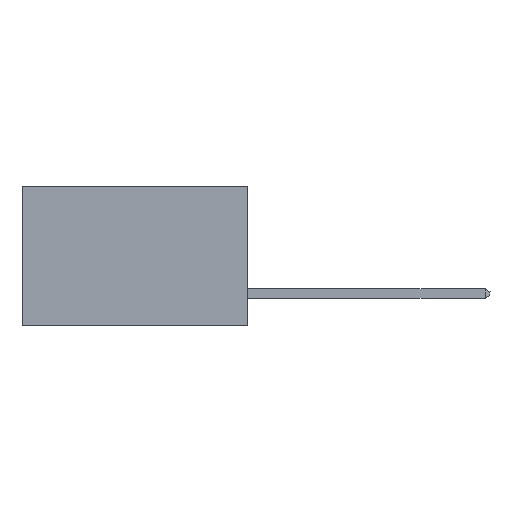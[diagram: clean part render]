
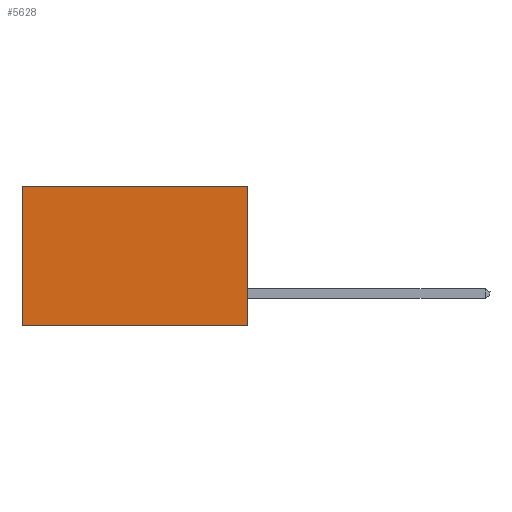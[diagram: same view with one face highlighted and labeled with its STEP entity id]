
A CAD part, left-side view. The second image highlights one B-rep face of the part: STEP entity #5628.
In plain terms, the highlighted planar face has unit normal (-1, 0, 0).
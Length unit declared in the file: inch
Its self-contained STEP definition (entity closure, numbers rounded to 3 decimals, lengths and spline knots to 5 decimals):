
#432 = CARTESIAN_POINT ( 'NONE',  ( 0.2615, 0.6, 0. ) ) ;
#1112 = VERTEX_POINT ( 'NONE', #9807 ) ;
#1156 = ORIENTED_EDGE ( 'NONE', *, *, #6772, .F. ) ;
#1478 = DIRECTION ( 'NONE',  ( 0., 1., 0. ) ) ;
#1571 = LINE ( 'NONE', #8122, #10280 ) ;
#1751 = VERTEX_POINT ( 'NONE', #432 ) ;
#2314 = FACE_OUTER_BOUND ( 'NONE', #3891, .T. ) ;
#2470 = ORIENTED_EDGE ( 'NONE', *, *, #9550, .T. ) ;
#3038 = EDGE_CURVE ( 'NONE', #3798, #1751, #3789, .T. ) ;
#3789 = LINE ( 'NONE', #7687, #6929 ) ;
#3798 = VERTEX_POINT ( 'NONE', #9347 ) ;
#3891 = EDGE_LOOP ( 'NONE', ( #2470, #1156, #8669, #4152 ) ) ;
#4152 = ORIENTED_EDGE ( 'NONE', *, *, #3038, .T. ) ;
#4418 = VERTEX_POINT ( 'NONE', #9647 ) ;
#4523 = DIRECTION ( 'NONE',  ( 0., 1., 0. ) ) ;
#4527 = CARTESIAN_POINT ( 'NONE',  ( 0.2615, 0., -0.37 ) ) ;
#4575 = DIRECTION ( 'NONE',  ( 1., 0., 0. ) ) ;
#4884 = DIRECTION ( 'NONE',  ( 0., 0., -1. ) ) ;
#5257 = LINE ( 'NONE', #5948, #5365 ) ;
#5365 = VECTOR ( 'NONE', #8401, 39.37008 ) ;
#5488 = VECTOR ( 'NONE', #1478, 39.37008 ) ;
#5628 = ADVANCED_FACE ( 'NONE', ( #2314 ), #6374, .F. ) ;
#5674 = CARTESIAN_POINT ( 'NONE',  ( 0.2615, 0., -0.37 ) ) ;
#5948 = CARTESIAN_POINT ( 'NONE',  ( 0.2615, 0.6, -0.37 ) ) ;
#6209 = DIRECTION ( 'NONE',  ( 0., 0., -1. ) ) ;
#6374 = PLANE ( 'NONE',  #9837 ) ;
#6377 = LINE ( 'NONE', #5674, #5488 ) ;
#6772 = EDGE_CURVE ( 'NONE', #4418, #1112, #6377, .T. ) ;
#6929 = VECTOR ( 'NONE', #4523, 39.37008 ) ;
#7687 = CARTESIAN_POINT ( 'NONE',  ( 0.2615, 0., 0. ) ) ;
#8122 = CARTESIAN_POINT ( 'NONE',  ( 0.2615, 0., -0.37 ) ) ;
#8401 = DIRECTION ( 'NONE',  ( 0., 0., -1. ) ) ;
#8669 = ORIENTED_EDGE ( 'NONE', *, *, #9779, .F. ) ;
#9347 = CARTESIAN_POINT ( 'NONE',  ( 0.2615, 0., 0. ) ) ;
#9550 = EDGE_CURVE ( 'NONE', #1751, #1112, #5257, .T. ) ;
#9647 = CARTESIAN_POINT ( 'NONE',  ( 0.2615, 0., -0.37 ) ) ;
#9779 = EDGE_CURVE ( 'NONE', #3798, #4418, #1571, .T. ) ;
#9807 = CARTESIAN_POINT ( 'NONE',  ( 0.2615, 0.6, -0.37 ) ) ;
#9837 = AXIS2_PLACEMENT_3D ( 'NONE', #4527, #4575, #6209 ) ;
#10280 = VECTOR ( 'NONE', #4884, 39.37008 ) ;
